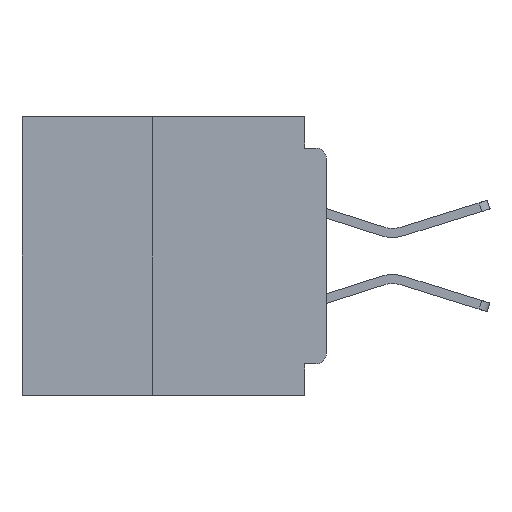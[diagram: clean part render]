
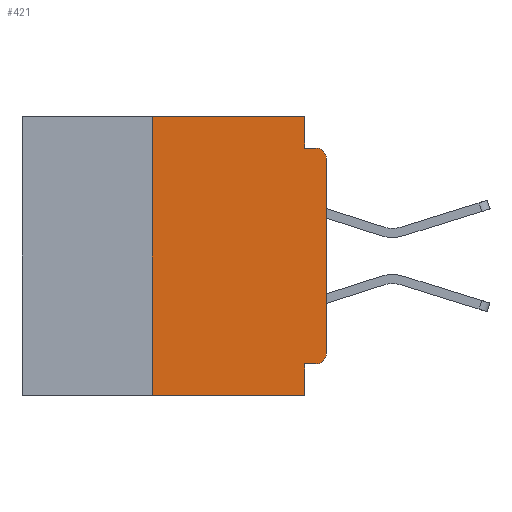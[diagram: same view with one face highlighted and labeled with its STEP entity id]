
A CAD part, left-side view. The second image highlights one B-rep face of the part: STEP entity #421.
In plain terms, the highlighted planar face has unit normal (-1, 0, 0).
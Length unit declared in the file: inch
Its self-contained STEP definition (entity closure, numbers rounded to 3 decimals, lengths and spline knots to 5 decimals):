
#18 = ORIENTED_EDGE ( 'NONE', *, *, #32763, .F. ) ;
#421 = ADVANCED_FACE ( 'NONE', ( #12109 ), #24775, .F. ) ;
#513 = LINE ( 'NONE', #2023, #18171 ) ;
#1013 = ORIENTED_EDGE ( 'NONE', *, *, #1902, .F. ) ;
#1902 = EDGE_CURVE ( 'NONE', #15280, #36180, #41154, .T. ) ;
#2023 = CARTESIAN_POINT ( 'NONE',  ( 0., 0., -0.355 ) ) ;
#2184 = DIRECTION ( 'NONE',  ( 0., 1., 0. ) ) ;
#3471 = CARTESIAN_POINT ( 'NONE',  ( 0., 0.031, 0. ) ) ;
#3816 = EDGE_CURVE ( 'NONE', #29418, #14480, #27345, .T. ) ;
#3900 = EDGE_CURVE ( 'NONE', #32584, #13862, #15482, .T. ) ;
#4167 = CARTESIAN_POINT ( 'NONE',  ( 0., 0.015, -0.355 ) ) ;
#4677 = DIRECTION ( 'NONE',  ( 0., -1., 0. ) ) ;
#5309 = ORIENTED_EDGE ( 'NONE', *, *, #3816, .T. ) ;
#6680 = VECTOR ( 'NONE', #19618, 39.37008 ) ;
#6728 = ORIENTED_EDGE ( 'NONE', *, *, #3900, .T. ) ;
#7611 = CARTESIAN_POINT ( 'NONE',  ( 0., 0.25, -0.4 ) ) ;
#8008 = CARTESIAN_POINT ( 'NONE',  ( 0., 0., -0.045 ) ) ;
#8359 = CARTESIAN_POINT ( 'NONE',  ( 0., 0.015, -0.34 ) ) ;
#9178 = CARTESIAN_POINT ( 'NONE',  ( 0., 0.25, -0.4 ) ) ;
#9193 = DIRECTION ( 'NONE',  ( 0., -1., 0. ) ) ;
#9462 = ORIENTED_EDGE ( 'NONE', *, *, #31938, .T. ) ;
#9636 = CARTESIAN_POINT ( 'NONE',  ( 0., 0.031, -0.4 ) ) ;
#10157 = AXIS2_PLACEMENT_3D ( 'NONE', #27755, #23677, #23523 ) ;
#10938 = DIRECTION ( 'NONE',  ( 0., 0., 1. ) ) ;
#11495 = CARTESIAN_POINT ( 'NONE',  ( 0., 0., 0. ) ) ;
#11672 = DIRECTION ( 'NONE',  ( 0., 0., -1. ) ) ;
#11695 = VERTEX_POINT ( 'NONE', #24743 ) ;
#12092 = ORIENTED_EDGE ( 'NONE', *, *, #37400, .F. ) ;
#12109 = FACE_OUTER_BOUND ( 'NONE', #15971, .T. ) ;
#12658 = CIRCLE ( 'NONE', #26245, 0.015 ) ;
#13006 = VECTOR ( 'NONE', #24625, 39.37008 ) ;
#13862 = VERTEX_POINT ( 'NONE', #9636 ) ;
#14167 = EDGE_CURVE ( 'NONE', #40498, #14480, #22625, .T. ) ;
#14480 = VERTEX_POINT ( 'NONE', #42252 ) ;
#15280 = VERTEX_POINT ( 'NONE', #27409 ) ;
#15482 = LINE ( 'NONE', #22746, #6680 ) ;
#15971 = EDGE_LOOP ( 'NONE', ( #34410, #5309, #39822, #21424, #1013, #12092, #6728, #18, #23468, #9462 ) ) ;
#16359 = VECTOR ( 'NONE', #10938, 39.37008 ) ;
#16677 = DIRECTION ( 'NONE',  ( 0., 0., -1. ) ) ;
#18100 = EDGE_CURVE ( 'NONE', #11695, #29418, #31490, .T. ) ;
#18171 = VECTOR ( 'NONE', #2184, 39.37008 ) ;
#19202 = DIRECTION ( 'NONE',  ( -1., 0., 0. ) ) ;
#19618 = DIRECTION ( 'NONE',  ( 0., -1., 0. ) ) ;
#20713 = DIRECTION ( 'NONE',  ( 0., 0., -1. ) ) ;
#21209 = EDGE_CURVE ( 'NONE', #36180, #40498, #26095, .T. ) ;
#21424 = ORIENTED_EDGE ( 'NONE', *, *, #21209, .F. ) ;
#21600 = VECTOR ( 'NONE', #4677, 39.37008 ) ;
#21872 = VERTEX_POINT ( 'NONE', #4167 ) ;
#22625 = LINE ( 'NONE', #8008, #21600 ) ;
#22746 = CARTESIAN_POINT ( 'NONE',  ( 0., 0.437, -0.4 ) ) ;
#23468 = ORIENTED_EDGE ( 'NONE', *, *, #41136, .F. ) ;
#23523 = DIRECTION ( 'NONE',  ( 0., 0., -1. ) ) ;
#23677 = DIRECTION ( 'NONE',  ( 1., 0., 0. ) ) ;
#23995 = LINE ( 'NONE', #32955, #39196 ) ;
#24625 = DIRECTION ( 'NONE',  ( 0., 0., 1. ) ) ;
#24743 = CARTESIAN_POINT ( 'NONE',  ( 0., 0., -0.34 ) ) ;
#24775 = PLANE ( 'NONE',  #10157 ) ;
#25140 = LINE ( 'NONE', #7611, #16359 ) ;
#26095 = LINE ( 'NONE', #40148, #42246 ) ;
#26245 = AXIS2_PLACEMENT_3D ( 'NONE', #8359, #31351, #11672 ) ;
#27345 = CIRCLE ( 'NONE', #32750, 0.015 ) ;
#27409 = CARTESIAN_POINT ( 'NONE',  ( 0., 0.25, 0. ) ) ;
#27755 = CARTESIAN_POINT ( 'NONE',  ( 0., 0.437, 0. ) ) ;
#29092 = CARTESIAN_POINT ( 'NONE',  ( 0., 0.031, -0.355 ) ) ;
#29418 = VERTEX_POINT ( 'NONE', #30864 ) ;
#30864 = CARTESIAN_POINT ( 'NONE',  ( 0., 0., -0.06 ) ) ;
#31351 = DIRECTION ( 'NONE',  ( -1., 0., 0. ) ) ;
#31490 = LINE ( 'NONE', #11495, #13006 ) ;
#31938 = EDGE_CURVE ( 'NONE', #21872, #11695, #12658, .T. ) ;
#32558 = VECTOR ( 'NONE', #9193, 39.37008 ) ;
#32584 = VERTEX_POINT ( 'NONE', #9178 ) ;
#32750 = AXIS2_PLACEMENT_3D ( 'NONE', #38648, #19202, #41880 ) ;
#32763 = EDGE_CURVE ( 'NONE', #35390, #13862, #23995, .T. ) ;
#32955 = CARTESIAN_POINT ( 'NONE',  ( 0., 0.031, -0.4 ) ) ;
#34410 = ORIENTED_EDGE ( 'NONE', *, *, #18100, .T. ) ;
#35390 = VERTEX_POINT ( 'NONE', #29092 ) ;
#36180 = VERTEX_POINT ( 'NONE', #3471 ) ;
#37400 = EDGE_CURVE ( 'NONE', #32584, #15280, #25140, .T. ) ;
#38502 = CARTESIAN_POINT ( 'NONE',  ( 0., 0.437, 0. ) ) ;
#38648 = CARTESIAN_POINT ( 'NONE',  ( 0., 0.015, -0.06 ) ) ;
#39196 = VECTOR ( 'NONE', #16677, 39.37008 ) ;
#39822 = ORIENTED_EDGE ( 'NONE', *, *, #14167, .F. ) ;
#40148 = CARTESIAN_POINT ( 'NONE',  ( 0., 0.031, 0. ) ) ;
#40498 = VERTEX_POINT ( 'NONE', #40883 ) ;
#40883 = CARTESIAN_POINT ( 'NONE',  ( 0., 0.031, -0.045 ) ) ;
#41136 = EDGE_CURVE ( 'NONE', #21872, #35390, #513, .T. ) ;
#41154 = LINE ( 'NONE', #38502, #32558 ) ;
#41880 = DIRECTION ( 'NONE',  ( 0., 0., -1. ) ) ;
#42246 = VECTOR ( 'NONE', #20713, 39.37008 ) ;
#42252 = CARTESIAN_POINT ( 'NONE',  ( 0., 0.015, -0.045 ) ) ;
